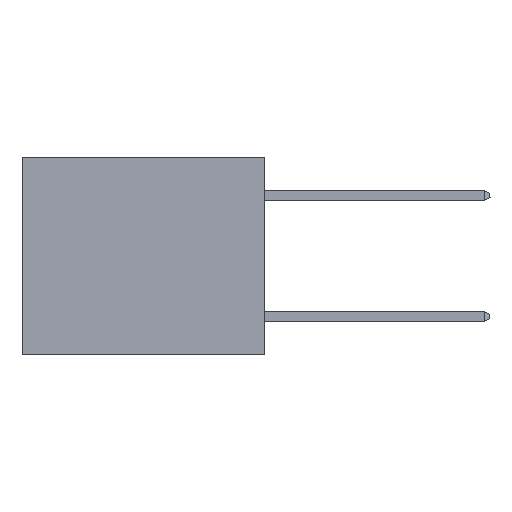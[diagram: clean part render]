
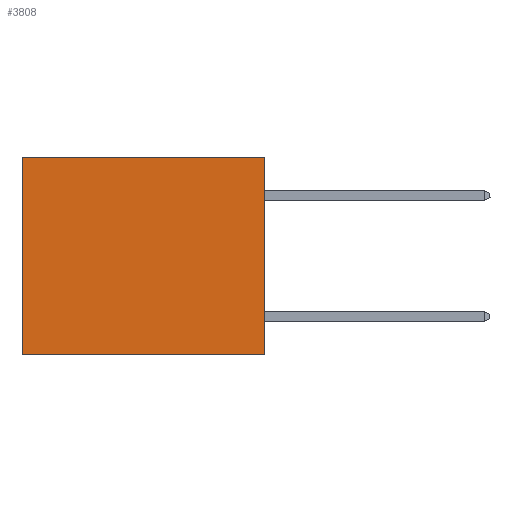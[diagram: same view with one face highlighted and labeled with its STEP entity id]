
A CAD part, left-side view. The second image highlights one B-rep face of the part: STEP entity #3808.
In plain terms, the highlighted planar face has unit normal (-1, 0, 0).
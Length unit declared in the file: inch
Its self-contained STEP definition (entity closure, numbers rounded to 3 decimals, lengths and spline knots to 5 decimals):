
#3808 = ADVANCED_FACE ( 'NONE', ( #13428 ), #19913, .F. ) ;
#3942 = CARTESIAN_POINT ( 'NONE',  ( 0.3165, 0., 0. ) ) ;
#4880 = EDGE_CURVE ( 'NONE', #9732, #15414, #26452, .T. ) ;
#5233 = EDGE_CURVE ( 'NONE', #9732, #23052, #24346, .T. ) ;
#6059 = CARTESIAN_POINT ( 'NONE',  ( 0.3165, 0.6, 0. ) ) ;
#6220 = VECTOR ( 'NONE', #15989, 39.37008 ) ;
#8376 = DIRECTION ( 'NONE',  ( 1., 0., 0. ) ) ;
#9732 = VERTEX_POINT ( 'NONE', #3942 ) ;
#10009 = CARTESIAN_POINT ( 'NONE',  ( 0.3165, 0., -0.49 ) ) ;
#10221 = EDGE_LOOP ( 'NONE', ( #12936, #22572, #22783, #26356 ) ) ;
#11414 = CARTESIAN_POINT ( 'NONE',  ( 0.3165, 0., 0. ) ) ;
#12699 = DIRECTION ( 'NONE',  ( 0., 0., -1. ) ) ;
#12936 = ORIENTED_EDGE ( 'NONE', *, *, #26772, .T. ) ;
#13297 = VERTEX_POINT ( 'NONE', #27735 ) ;
#13428 = FACE_OUTER_BOUND ( 'NONE', #10221, .T. ) ;
#13863 = VECTOR ( 'NONE', #28701, 39.37008 ) ;
#14870 = CARTESIAN_POINT ( 'NONE',  ( 0.3165, 0.6, -0.49 ) ) ;
#14932 = LINE ( 'NONE', #14870, #13863 ) ;
#15228 = CARTESIAN_POINT ( 'NONE',  ( 0.3165, 0., -0.49 ) ) ;
#15414 = VERTEX_POINT ( 'NONE', #20521 ) ;
#15989 = DIRECTION ( 'NONE',  ( 0., 1., 0. ) ) ;
#16580 = CARTESIAN_POINT ( 'NONE',  ( 0.3165, 0., -0.49 ) ) ;
#18620 = AXIS2_PLACEMENT_3D ( 'NONE', #15228, #8376, #26692 ) ;
#18773 = LINE ( 'NONE', #10009, #26863 ) ;
#19913 = PLANE ( 'NONE',  #18620 ) ;
#20521 = CARTESIAN_POINT ( 'NONE',  ( 0.3165, 0., -0.49 ) ) ;
#22572 = ORIENTED_EDGE ( 'NONE', *, *, #27858, .F. ) ;
#22783 = ORIENTED_EDGE ( 'NONE', *, *, #4880, .F. ) ;
#23052 = VERTEX_POINT ( 'NONE', #6059 ) ;
#23519 = DIRECTION ( 'NONE',  ( 0., 1., 0. ) ) ;
#24346 = LINE ( 'NONE', #11414, #6220 ) ;
#25059 = VECTOR ( 'NONE', #12699, 39.37008 ) ;
#26356 = ORIENTED_EDGE ( 'NONE', *, *, #5233, .T. ) ;
#26452 = LINE ( 'NONE', #16580, #25059 ) ;
#26692 = DIRECTION ( 'NONE',  ( 0., 0., -1. ) ) ;
#26772 = EDGE_CURVE ( 'NONE', #23052, #13297, #14932, .T. ) ;
#26863 = VECTOR ( 'NONE', #23519, 39.37008 ) ;
#27735 = CARTESIAN_POINT ( 'NONE',  ( 0.3165, 0.6, -0.49 ) ) ;
#27858 = EDGE_CURVE ( 'NONE', #15414, #13297, #18773, .T. ) ;
#28701 = DIRECTION ( 'NONE',  ( 0., 0., -1. ) ) ;
